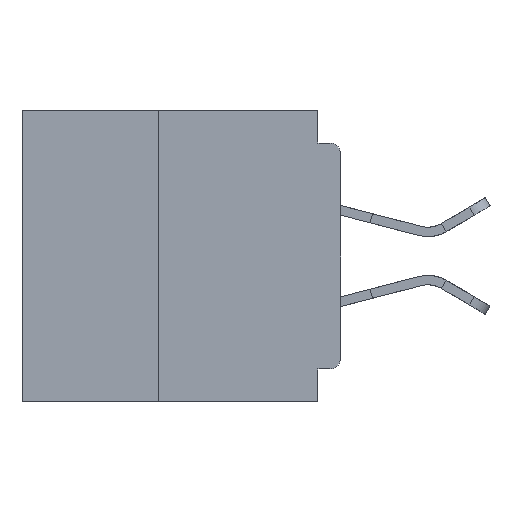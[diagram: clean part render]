
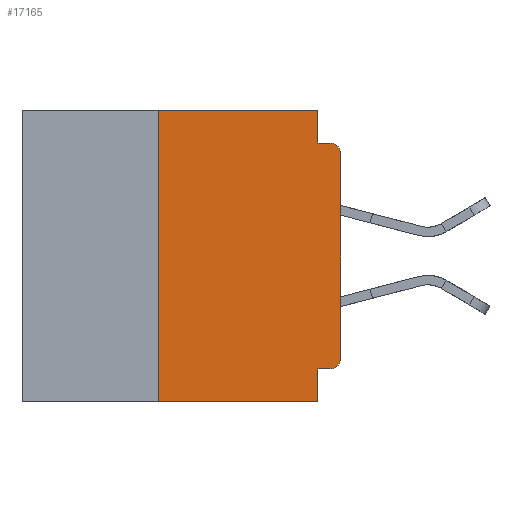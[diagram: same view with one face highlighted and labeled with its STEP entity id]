
A CAD part, left-side view. The second image highlights one B-rep face of the part: STEP entity #17165.
In plain terms, the highlighted planar face has unit normal (-1, 0, 0).
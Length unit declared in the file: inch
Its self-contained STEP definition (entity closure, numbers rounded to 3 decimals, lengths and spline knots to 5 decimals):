
#305 = AXIS2_PLACEMENT_3D ( 'NONE', #25374, #32005, #12270 ) ;
#754 = VECTOR ( 'NONE', #3419, 39.37008 ) ;
#1065 = VERTEX_POINT ( 'NONE', #29272 ) ;
#1322 = ORIENTED_EDGE ( 'NONE', *, *, #23393, .F. ) ;
#1374 = CARTESIAN_POINT ( 'NONE',  ( 0., 0.031, -0.4 ) ) ;
#1489 = DIRECTION ( 'NONE',  ( 0., 0., 1. ) ) ;
#1632 = ORIENTED_EDGE ( 'NONE', *, *, #2985, .T. ) ;
#2231 = CARTESIAN_POINT ( 'NONE',  ( 0., 0., -0.06 ) ) ;
#2766 = DIRECTION ( 'NONE',  ( 0., 1., 0. ) ) ;
#2985 = EDGE_CURVE ( 'NONE', #38394, #41313, #19855, .T. ) ;
#3270 = CARTESIAN_POINT ( 'NONE',  ( 0., 0., -0.34 ) ) ;
#3419 = DIRECTION ( 'NONE',  ( 0., -1., 0. ) ) ;
#3799 = LINE ( 'NONE', #24598, #29099 ) ;
#4106 = VERTEX_POINT ( 'NONE', #38101 ) ;
#4365 = AXIS2_PLACEMENT_3D ( 'NONE', #11048, #34078, #14323 ) ;
#6289 = EDGE_CURVE ( 'NONE', #11380, #7487, #31546, .T. ) ;
#6907 = EDGE_CURVE ( 'NONE', #1065, #38394, #40779, .T. ) ;
#7278 = DIRECTION ( 'NONE',  ( 0., -1., 0. ) ) ;
#7487 = VERTEX_POINT ( 'NONE', #21184 ) ;
#8255 = LINE ( 'NONE', #32373, #34519 ) ;
#8431 = ORIENTED_EDGE ( 'NONE', *, *, #29385, .T. ) ;
#9425 = ORIENTED_EDGE ( 'NONE', *, *, #6907, .T. ) ;
#9604 = LINE ( 'NONE', #13262, #754 ) ;
#9798 = ORIENTED_EDGE ( 'NONE', *, *, #38409, .F. ) ;
#10004 = ORIENTED_EDGE ( 'NONE', *, *, #24605, .F. ) ;
#10977 = CARTESIAN_POINT ( 'NONE',  ( 0., 0.031, 0. ) ) ;
#11048 = CARTESIAN_POINT ( 'NONE',  ( 0., 0.015, -0.06 ) ) ;
#11380 = VERTEX_POINT ( 'NONE', #27337 ) ;
#11482 = VERTEX_POINT ( 'NONE', #41172 ) ;
#11791 = LINE ( 'NONE', #26987, #29281 ) ;
#11929 = CARTESIAN_POINT ( 'NONE',  ( 0., 0.015, -0.34 ) ) ;
#11952 = DIRECTION ( 'NONE',  ( 0., 0., 1. ) ) ;
#12085 = EDGE_LOOP ( 'NONE', ( #1632, #26076, #9798, #1322, #10004, #34677, #8431, #34037, #21622, #9425 ) ) ;
#12270 = DIRECTION ( 'NONE',  ( 0., 0., -1. ) ) ;
#12287 = LINE ( 'NONE', #40198, #29773 ) ;
#12978 = VECTOR ( 'NONE', #27947, 39.37008 ) ;
#13262 = CARTESIAN_POINT ( 'NONE',  ( 0., 0., -0.045 ) ) ;
#14149 = VERTEX_POINT ( 'NONE', #28079 ) ;
#14323 = DIRECTION ( 'NONE',  ( 0., 0., -1. ) ) ;
#15203 = DIRECTION ( 'NONE',  ( 0., 0., -1. ) ) ;
#17165 = ADVANCED_FACE ( 'NONE', ( #25354 ), #41813, .F. ) ;
#17193 = VERTEX_POINT ( 'NONE', #28818 ) ;
#19855 = LINE ( 'NONE', #35114, #36377 ) ;
#20395 = DIRECTION ( 'NONE',  ( 0., -1., 0. ) ) ;
#20473 = AXIS2_PLACEMENT_3D ( 'NONE', #11929, #34948, #15203 ) ;
#21184 = CARTESIAN_POINT ( 'NONE',  ( 0., 0.031, -0.4 ) ) ;
#21622 = ORIENTED_EDGE ( 'NONE', *, *, #33875, .F. ) ;
#21996 = CIRCLE ( 'NONE', #4365, 0.015 ) ;
#23393 = EDGE_CURVE ( 'NONE', #17193, #11482, #42244, .T. ) ;
#24598 = CARTESIAN_POINT ( 'NONE',  ( 0., 0.25, -0.4 ) ) ;
#24605 = EDGE_CURVE ( 'NONE', #4106, #17193, #11791, .T. ) ;
#25244 = EDGE_CURVE ( 'NONE', #41313, #14149, #21996, .T. ) ;
#25354 = FACE_OUTER_BOUND ( 'NONE', #12085, .T. ) ;
#25374 = CARTESIAN_POINT ( 'NONE',  ( 0., 0.437, 0. ) ) ;
#26076 = ORIENTED_EDGE ( 'NONE', *, *, #25244, .T. ) ;
#26987 = CARTESIAN_POINT ( 'NONE',  ( 0., 0.437, 0. ) ) ;
#27337 = CARTESIAN_POINT ( 'NONE',  ( 0., 0.031, -0.355 ) ) ;
#27947 = DIRECTION ( 'NONE',  ( 0., 0., -1. ) ) ;
#28079 = CARTESIAN_POINT ( 'NONE',  ( 0., 0.015, -0.045 ) ) ;
#28818 = CARTESIAN_POINT ( 'NONE',  ( 0., 0.031, 0. ) ) ;
#29099 = VECTOR ( 'NONE', #1489, 39.37008 ) ;
#29272 = CARTESIAN_POINT ( 'NONE',  ( 0., 0.015, -0.355 ) ) ;
#29281 = VECTOR ( 'NONE', #7278, 39.37008 ) ;
#29385 = EDGE_CURVE ( 'NONE', #32777, #7487, #12287, .T. ) ;
#29513 = CARTESIAN_POINT ( 'NONE',  ( 0., 0.25, -0.4 ) ) ;
#29773 = VECTOR ( 'NONE', #20395, 39.37008 ) ;
#31546 = LINE ( 'NONE', #1374, #12978 ) ;
#32005 = DIRECTION ( 'NONE',  ( 1., 0., 0. ) ) ;
#32373 = CARTESIAN_POINT ( 'NONE',  ( 0., 0., -0.355 ) ) ;
#32777 = VERTEX_POINT ( 'NONE', #29513 ) ;
#33875 = EDGE_CURVE ( 'NONE', #1065, #11380, #8255, .T. ) ;
#34037 = ORIENTED_EDGE ( 'NONE', *, *, #6289, .F. ) ;
#34078 = DIRECTION ( 'NONE',  ( -1., 0., 0. ) ) ;
#34519 = VECTOR ( 'NONE', #2766, 39.37008 ) ;
#34677 = ORIENTED_EDGE ( 'NONE', *, *, #39228, .F. ) ;
#34948 = DIRECTION ( 'NONE',  ( -1., 0., 0. ) ) ;
#35114 = CARTESIAN_POINT ( 'NONE',  ( 0., 0., 0. ) ) ;
#36377 = VECTOR ( 'NONE', #11952, 39.37008 ) ;
#37337 = DIRECTION ( 'NONE',  ( 0., 0., -1. ) ) ;
#38101 = CARTESIAN_POINT ( 'NONE',  ( 0., 0.25, 0. ) ) ;
#38394 = VERTEX_POINT ( 'NONE', #3270 ) ;
#38409 = EDGE_CURVE ( 'NONE', #11482, #14149, #9604, .T. ) ;
#39136 = VECTOR ( 'NONE', #37337, 39.37008 ) ;
#39228 = EDGE_CURVE ( 'NONE', #32777, #4106, #3799, .T. ) ;
#40198 = CARTESIAN_POINT ( 'NONE',  ( 0., 0.437, -0.4 ) ) ;
#40779 = CIRCLE ( 'NONE', #20473, 0.015 ) ;
#41172 = CARTESIAN_POINT ( 'NONE',  ( 0., 0.031, -0.045 ) ) ;
#41313 = VERTEX_POINT ( 'NONE', #2231 ) ;
#41813 = PLANE ( 'NONE',  #305 ) ;
#42244 = LINE ( 'NONE', #10977, #39136 ) ;
